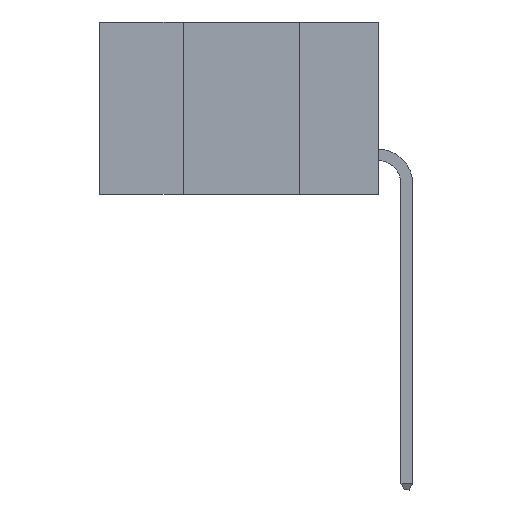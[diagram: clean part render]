
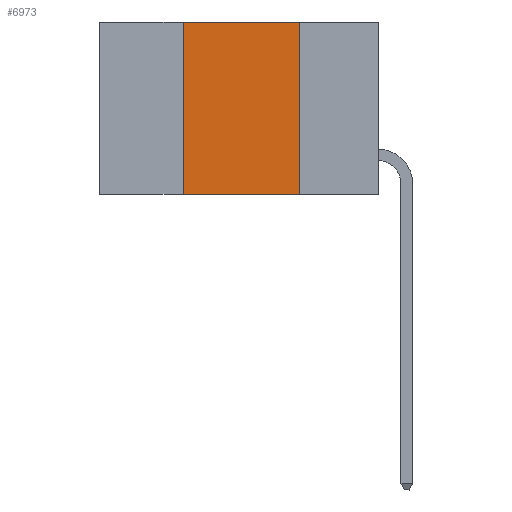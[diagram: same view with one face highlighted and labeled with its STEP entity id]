
A CAD part, left-side view. The second image highlights one B-rep face of the part: STEP entity #6973.
In plain terms, the highlighted planar face has unit normal (-1, 0, 0).
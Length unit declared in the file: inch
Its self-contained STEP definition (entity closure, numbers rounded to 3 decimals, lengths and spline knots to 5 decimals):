
#212 = DIRECTION ( 'NONE',  ( 0., 0., -1. ) ) ;
#324 = CARTESIAN_POINT ( 'NONE',  ( 0., 0.17, -0.37 ) ) ;
#374 = EDGE_CURVE ( 'NONE', #7672, #2059, #6361, .T. ) ;
#1043 = CARTESIAN_POINT ( 'NONE',  ( 0., 0.17, 0. ) ) ;
#1269 = LINE ( 'NONE', #3271, #7507 ) ;
#1304 = FACE_OUTER_BOUND ( 'NONE', #10245, .T. ) ;
#1861 = ORIENTED_EDGE ( 'NONE', *, *, #2238, .F. ) ;
#2059 = VERTEX_POINT ( 'NONE', #7966 ) ;
#2195 = ORIENTED_EDGE ( 'NONE', *, *, #374, .F. ) ;
#2238 = EDGE_CURVE ( 'NONE', #8827, #3578, #6502, .T. ) ;
#2529 = ORIENTED_EDGE ( 'NONE', *, *, #3162, .F. ) ;
#3162 = EDGE_CURVE ( 'NONE', #2059, #8827, #1269, .T. ) ;
#3271 = CARTESIAN_POINT ( 'NONE',  ( 0., 0.6, 0. ) ) ;
#3578 = VERTEX_POINT ( 'NONE', #324 ) ;
#3719 = CARTESIAN_POINT ( 'NONE',  ( 0., 0.6, 0. ) ) ;
#4013 = DIRECTION ( 'NONE',  ( 0., -1., 0. ) ) ;
#4378 = ORIENTED_EDGE ( 'NONE', *, *, #7361, .T. ) ;
#4678 = DIRECTION ( 'NONE',  ( 0., 0., 1. ) ) ;
#4739 = DIRECTION ( 'NONE',  ( 0., -1., 0. ) ) ;
#5250 = VECTOR ( 'NONE', #4739, 39.37008 ) ;
#5480 = CARTESIAN_POINT ( 'NONE',  ( 0., 0.6, -0.37 ) ) ;
#6361 = LINE ( 'NONE', #7101, #9382 ) ;
#6502 = LINE ( 'NONE', #1043, #9922 ) ;
#6973 = ADVANCED_FACE ( 'NONE', ( #1304 ), #10352, .F. ) ;
#7043 = DIRECTION ( 'NONE',  ( 1., 0., 0. ) ) ;
#7101 = CARTESIAN_POINT ( 'NONE',  ( 0., 0.42, 0. ) ) ;
#7361 = EDGE_CURVE ( 'NONE', #7672, #3578, #9808, .T. ) ;
#7507 = VECTOR ( 'NONE', #4013, 39.37008 ) ;
#7672 = VERTEX_POINT ( 'NONE', #9207 ) ;
#7963 = CARTESIAN_POINT ( 'NONE',  ( 0., 0.17, 0. ) ) ;
#7966 = CARTESIAN_POINT ( 'NONE',  ( 0., 0.42, 0. ) ) ;
#8686 = DIRECTION ( 'NONE',  ( 0., 0., -1. ) ) ;
#8827 = VERTEX_POINT ( 'NONE', #7963 ) ;
#9207 = CARTESIAN_POINT ( 'NONE',  ( 0., 0.42, -0.37 ) ) ;
#9257 = AXIS2_PLACEMENT_3D ( 'NONE', #3719, #7043, #8686 ) ;
#9382 = VECTOR ( 'NONE', #4678, 39.37008 ) ;
#9808 = LINE ( 'NONE', #5480, #5250 ) ;
#9922 = VECTOR ( 'NONE', #212, 39.37008 ) ;
#10245 = EDGE_LOOP ( 'NONE', ( #1861, #2529, #2195, #4378 ) ) ;
#10352 = PLANE ( 'NONE',  #9257 ) ;
